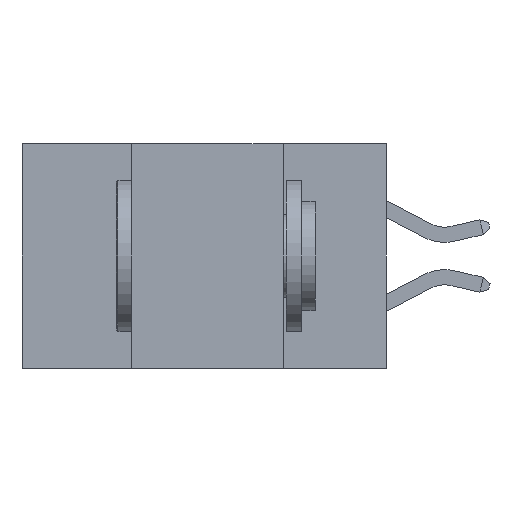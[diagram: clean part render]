
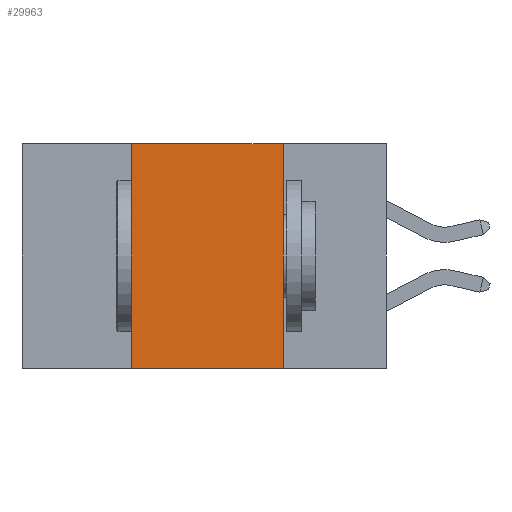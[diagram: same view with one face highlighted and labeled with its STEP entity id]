
A CAD part, left-side view. The second image highlights one B-rep face of the part: STEP entity #29963.
In plain terms, the highlighted planar face has unit normal (-1, 0, 0).
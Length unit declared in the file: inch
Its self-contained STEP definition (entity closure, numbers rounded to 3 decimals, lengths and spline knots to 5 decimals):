
#1351 = CARTESIAN_POINT ( 'NONE',  ( 0., 0.6, -0.37 ) ) ;
#3199 = CARTESIAN_POINT ( 'NONE',  ( 0., 0.6, 0. ) ) ;
#5728 = VERTEX_POINT ( 'NONE', #7623 ) ;
#7623 = CARTESIAN_POINT ( 'NONE',  ( 0., 0.17, 0. ) ) ;
#8777 = DIRECTION ( 'NONE',  ( 0., 0., -1. ) ) ;
#9299 = EDGE_CURVE ( 'NONE', #16845, #26430, #31721, .T. ) ;
#10434 = VECTOR ( 'NONE', #13860, 39.37008 ) ;
#10574 = ORIENTED_EDGE ( 'NONE', *, *, #33701, .F. ) ;
#11291 = DIRECTION ( 'NONE',  ( 0., -1., 0. ) ) ;
#12113 = FACE_OUTER_BOUND ( 'NONE', #26034, .T. ) ;
#13327 = LINE ( 'NONE', #1351, #15833 ) ;
#13757 = LINE ( 'NONE', #14086, #19998 ) ;
#13860 = DIRECTION ( 'NONE',  ( 0., -1., 0. ) ) ;
#14086 = CARTESIAN_POINT ( 'NONE',  ( 0., 0.17, 0. ) ) ;
#14287 = CARTESIAN_POINT ( 'NONE',  ( 0., 0.42, 0. ) ) ;
#15430 = VERTEX_POINT ( 'NONE', #27698 ) ;
#15833 = VECTOR ( 'NONE', #11291, 39.37008 ) ;
#16022 = DIRECTION ( 'NONE',  ( 0., 0., 1. ) ) ;
#16498 = DIRECTION ( 'NONE',  ( 1., 0., 0. ) ) ;
#16741 = PLANE ( 'NONE',  #26966 ) ;
#16845 = VERTEX_POINT ( 'NONE', #22128 ) ;
#17711 = VECTOR ( 'NONE', #16022, 39.37008 ) ;
#19536 = CARTESIAN_POINT ( 'NONE',  ( 0., 0.6, 0. ) ) ;
#19992 = LINE ( 'NONE', #3199, #10434 ) ;
#19998 = VECTOR ( 'NONE', #24399, 39.37008 ) ;
#22128 = CARTESIAN_POINT ( 'NONE',  ( 0., 0.42, -0.37 ) ) ;
#24399 = DIRECTION ( 'NONE',  ( 0., 0., -1. ) ) ;
#24840 = EDGE_CURVE ( 'NONE', #16845, #15430, #13327, .T. ) ;
#25643 = ORIENTED_EDGE ( 'NONE', *, *, #24840, .T. ) ;
#25656 = EDGE_CURVE ( 'NONE', #26430, #5728, #19992, .T. ) ;
#26034 = EDGE_LOOP ( 'NONE', ( #10574, #30081, #28617, #25643 ) ) ;
#26430 = VERTEX_POINT ( 'NONE', #14287 ) ;
#26496 = CARTESIAN_POINT ( 'NONE',  ( 0., 0.42, 0. ) ) ;
#26966 = AXIS2_PLACEMENT_3D ( 'NONE', #19536, #16498, #8777 ) ;
#27698 = CARTESIAN_POINT ( 'NONE',  ( 0., 0.17, -0.37 ) ) ;
#28617 = ORIENTED_EDGE ( 'NONE', *, *, #9299, .F. ) ;
#29963 = ADVANCED_FACE ( 'NONE', ( #12113 ), #16741, .F. ) ;
#30081 = ORIENTED_EDGE ( 'NONE', *, *, #25656, .F. ) ;
#31721 = LINE ( 'NONE', #26496, #17711 ) ;
#33701 = EDGE_CURVE ( 'NONE', #5728, #15430, #13757, .T. ) ;
